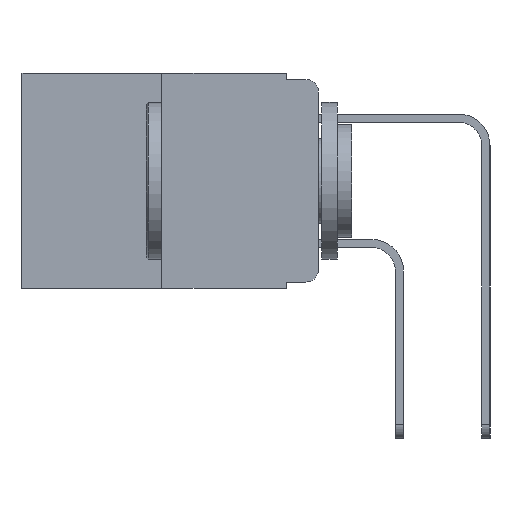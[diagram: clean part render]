
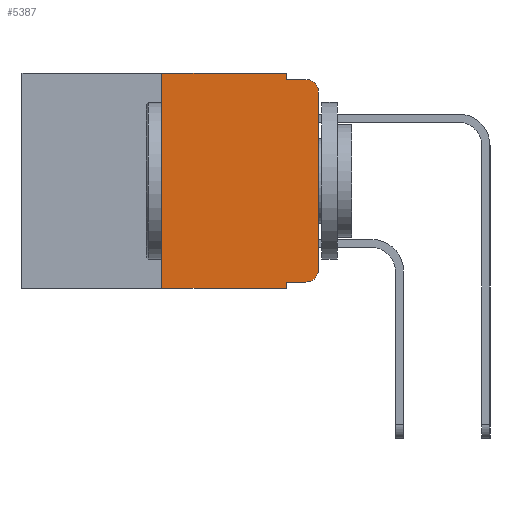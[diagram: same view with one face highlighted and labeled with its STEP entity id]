
A CAD part, left-side view. The second image highlights one B-rep face of the part: STEP entity #5387.
In plain terms, the highlighted planar face has unit normal (-1, 0, 0).
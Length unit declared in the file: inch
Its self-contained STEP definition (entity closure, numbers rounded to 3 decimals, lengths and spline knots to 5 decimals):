
#243 = CARTESIAN_POINT ( 'NONE',  ( 0., 0.25, 0. ) ) ;
#370 = DIRECTION ( 'NONE',  ( 0., -1., 0. ) ) ;
#514 = DIRECTION ( 'NONE',  ( 0., 0., -1. ) ) ;
#854 = CARTESIAN_POINT ( 'NONE',  ( 0., 0.051, 0. ) ) ;
#882 = DIRECTION ( 'NONE',  ( -1., 0., 0. ) ) ;
#988 = AXIS2_PLACEMENT_3D ( 'NONE', #19096, #2631, #13339 ) ;
#1057 = EDGE_CURVE ( 'NONE', #13440, #8562, #10874, .T. ) ;
#1432 = AXIS2_PLACEMENT_3D ( 'NONE', #6852, #17224, #8358 ) ;
#2143 = EDGE_CURVE ( 'NONE', #5306, #13440, #15748, .T. ) ;
#2232 = ORIENTED_EDGE ( 'NONE', *, *, #5343, .F. ) ;
#2631 = DIRECTION ( 'NONE',  ( 1., 0., 0. ) ) ;
#2667 = VERTEX_POINT ( 'NONE', #19057 ) ;
#2751 = FACE_OUTER_BOUND ( 'NONE', #11768, .T. ) ;
#3087 = CARTESIAN_POINT ( 'NONE',  ( 0., 0., 0. ) ) ;
#3224 = EDGE_CURVE ( 'NONE', #5306, #7957, #6564, .T. ) ;
#3247 = VECTOR ( 'NONE', #14684, 39.37008 ) ;
#3487 = CARTESIAN_POINT ( 'NONE',  ( 0., 0.02, -0.333 ) ) ;
#3655 = CARTESIAN_POINT ( 'NONE',  ( 0., 0., -0.03 ) ) ;
#3749 = ORIENTED_EDGE ( 'NONE', *, *, #2143, .T. ) ;
#3772 = EDGE_CURVE ( 'NONE', #5024, #4048, #4073, .T. ) ;
#4048 = VERTEX_POINT ( 'NONE', #7339 ) ;
#4073 = LINE ( 'NONE', #17142, #19450 ) ;
#4271 = EDGE_CURVE ( 'NONE', #2667, #5024, #10758, .T. ) ;
#5024 = VERTEX_POINT ( 'NONE', #12311 ) ;
#5306 = VERTEX_POINT ( 'NONE', #5554 ) ;
#5343 = EDGE_CURVE ( 'NONE', #4048, #16706, #11876, .T. ) ;
#5387 = ADVANCED_FACE ( 'NONE', ( #2751 ), #5744, .F. ) ;
#5554 = CARTESIAN_POINT ( 'NONE',  ( 0., 0.051, -0.333 ) ) ;
#5744 = PLANE ( 'NONE',  #988 ) ;
#6071 = VECTOR ( 'NONE', #11458, 39.37008 ) ;
#6249 = VERTEX_POINT ( 'NONE', #3655 ) ;
#6395 = EDGE_CURVE ( 'NONE', #16706, #16886, #7431, .T. ) ;
#6448 = ORIENTED_EDGE ( 'NONE', *, *, #3772, .F. ) ;
#6564 = LINE ( 'NONE', #14891, #6071 ) ;
#6852 = CARTESIAN_POINT ( 'NONE',  ( 0., 0.02, -0.03 ) ) ;
#6942 = ORIENTED_EDGE ( 'NONE', *, *, #4271, .F. ) ;
#7339 = CARTESIAN_POINT ( 'NONE',  ( 0., 0.051, 0. ) ) ;
#7427 = ORIENTED_EDGE ( 'NONE', *, *, #3224, .F. ) ;
#7431 = LINE ( 'NONE', #11665, #3247 ) ;
#7437 = EDGE_CURVE ( 'NONE', #6249, #16886, #7847, .T. ) ;
#7699 = CARTESIAN_POINT ( 'NONE',  ( 0., 0.02, -0.01 ) ) ;
#7847 = CIRCLE ( 'NONE', #1432, 0.02 ) ;
#7957 = VERTEX_POINT ( 'NONE', #14001 ) ;
#8007 = VECTOR ( 'NONE', #370, 39.37008 ) ;
#8358 = DIRECTION ( 'NONE',  ( 0., 0., -1. ) ) ;
#8423 = EDGE_CURVE ( 'NONE', #8562, #6249, #15288, .T. ) ;
#8562 = VERTEX_POINT ( 'NONE', #14054 ) ;
#9373 = CARTESIAN_POINT ( 'NONE',  ( 0., 0.051, -0.333 ) ) ;
#9998 = DIRECTION ( 'NONE',  ( 0., 0., 1. ) ) ;
#10758 = LINE ( 'NONE', #243, #18555 ) ;
#10838 = VECTOR ( 'NONE', #15268, 39.37008 ) ;
#10874 = CIRCLE ( 'NONE', #11086, 0.02 ) ;
#10882 = DIRECTION ( 'NONE',  ( 0., -1., 0. ) ) ;
#11086 = AXIS2_PLACEMENT_3D ( 'NONE', #14475, #882, #514 ) ;
#11416 = VECTOR ( 'NONE', #13207, 39.37008 ) ;
#11458 = DIRECTION ( 'NONE',  ( 0., 0., -1. ) ) ;
#11665 = CARTESIAN_POINT ( 'NONE',  ( 0., 0.051, -0.01 ) ) ;
#11768 = EDGE_LOOP ( 'NONE', ( #13036, #13500, #17365, #2232, #6448, #6942, #14904, #7427, #3749, #19597 ) ) ;
#11815 = CARTESIAN_POINT ( 'NONE',  ( 0., 0.051, -0.01 ) ) ;
#11876 = LINE ( 'NONE', #854, #11416 ) ;
#12311 = CARTESIAN_POINT ( 'NONE',  ( 0., 0.25, 0. ) ) ;
#13036 = ORIENTED_EDGE ( 'NONE', *, *, #8423, .T. ) ;
#13207 = DIRECTION ( 'NONE',  ( 0., 0., -1. ) ) ;
#13339 = DIRECTION ( 'NONE',  ( 0., 0., -1. ) ) ;
#13440 = VERTEX_POINT ( 'NONE', #3487 ) ;
#13500 = ORIENTED_EDGE ( 'NONE', *, *, #7437, .T. ) ;
#14001 = CARTESIAN_POINT ( 'NONE',  ( 0., 0.051, -0.343 ) ) ;
#14054 = CARTESIAN_POINT ( 'NONE',  ( 0., 0., -0.313 ) ) ;
#14107 = EDGE_CURVE ( 'NONE', #2667, #7957, #19258, .T. ) ;
#14260 = DIRECTION ( 'NONE',  ( 0., -1., 0. ) ) ;
#14475 = CARTESIAN_POINT ( 'NONE',  ( 0., 0.02, -0.313 ) ) ;
#14684 = DIRECTION ( 'NONE',  ( 0., -1., 0. ) ) ;
#14891 = CARTESIAN_POINT ( 'NONE',  ( 0., 0.051, 0. ) ) ;
#14904 = ORIENTED_EDGE ( 'NONE', *, *, #14107, .T. ) ;
#15268 = DIRECTION ( 'NONE',  ( 0., 0., 1. ) ) ;
#15288 = LINE ( 'NONE', #3087, #10838 ) ;
#15301 = VECTOR ( 'NONE', #10882, 39.37008 ) ;
#15748 = LINE ( 'NONE', #9373, #15301 ) ;
#16706 = VERTEX_POINT ( 'NONE', #11815 ) ;
#16886 = VERTEX_POINT ( 'NONE', #7699 ) ;
#17142 = CARTESIAN_POINT ( 'NONE',  ( 0., 0.473, 0. ) ) ;
#17224 = DIRECTION ( 'NONE',  ( -1., 0., 0. ) ) ;
#17365 = ORIENTED_EDGE ( 'NONE', *, *, #6395, .F. ) ;
#18555 = VECTOR ( 'NONE', #9998, 39.37008 ) ;
#18574 = CARTESIAN_POINT ( 'NONE',  ( 0., 0.473, -0.343 ) ) ;
#19057 = CARTESIAN_POINT ( 'NONE',  ( 0., 0.25, -0.343 ) ) ;
#19096 = CARTESIAN_POINT ( 'NONE',  ( 0., 0.473, 0. ) ) ;
#19258 = LINE ( 'NONE', #18574, #8007 ) ;
#19450 = VECTOR ( 'NONE', #14260, 39.37008 ) ;
#19597 = ORIENTED_EDGE ( 'NONE', *, *, #1057, .T. ) ;
